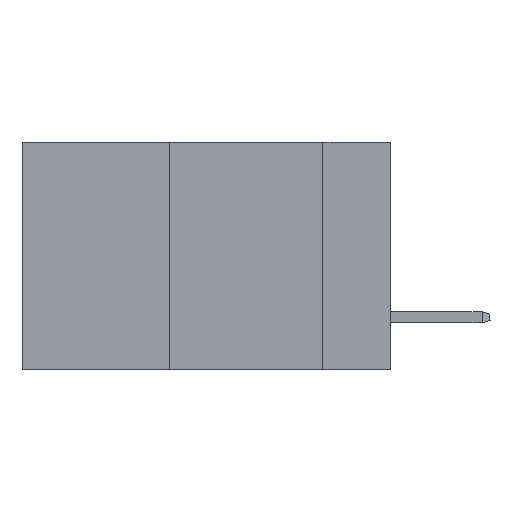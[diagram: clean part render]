
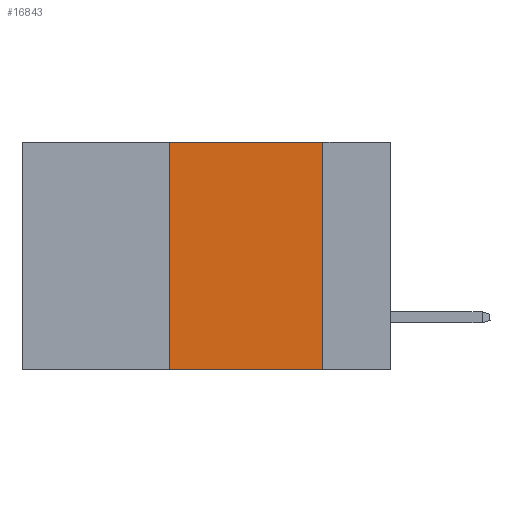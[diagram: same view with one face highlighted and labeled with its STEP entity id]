
A CAD part, left-side view. The second image highlights one B-rep face of the part: STEP entity #16843.
In plain terms, the highlighted planar face has unit normal (-1, 0, 0).
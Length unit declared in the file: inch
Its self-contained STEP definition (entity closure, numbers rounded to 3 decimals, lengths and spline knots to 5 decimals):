
#369 = EDGE_CURVE ( 'NONE', #24583, #14350, #24584, .T. ) ;
#1089 = VERTEX_POINT ( 'NONE', #12770 ) ;
#2658 = DIRECTION ( 'NONE',  ( 1., 0., 0. ) ) ;
#2930 = DIRECTION ( 'NONE',  ( 0., 0., -1. ) ) ;
#3265 = DIRECTION ( 'NONE',  ( 0., 0., 1. ) ) ;
#3415 = EDGE_LOOP ( 'NONE', ( #5046, #25634, #13580, #16845 ) ) ;
#3771 = CARTESIAN_POINT ( 'NONE',  ( 0., 0.6, -0.37 ) ) ;
#5046 = ORIENTED_EDGE ( 'NONE', *, *, #12262, .F. ) ;
#5700 = VECTOR ( 'NONE', #8270, 39.37008 ) ;
#7971 = LINE ( 'NONE', #13589, #9642 ) ;
#8270 = DIRECTION ( 'NONE',  ( 0., -1., 0. ) ) ;
#8736 = FACE_OUTER_BOUND ( 'NONE', #3415, .T. ) ;
#9524 = VERTEX_POINT ( 'NONE', #24870 ) ;
#9642 = VECTOR ( 'NONE', #20105, 39.37008 ) ;
#12262 = EDGE_CURVE ( 'NONE', #14350, #1089, #7971, .T. ) ;
#12770 = CARTESIAN_POINT ( 'NONE',  ( 0., 0.11, -0.37 ) ) ;
#13580 = ORIENTED_EDGE ( 'NONE', *, *, #20589, .F. ) ;
#13589 = CARTESIAN_POINT ( 'NONE',  ( 0., 0.11, 0. ) ) ;
#14350 = VERTEX_POINT ( 'NONE', #20264 ) ;
#15600 = CARTESIAN_POINT ( 'NONE',  ( 0., 0.6, 0. ) ) ;
#15626 = LINE ( 'NONE', #24639, #22579 ) ;
#16843 = ADVANCED_FACE ( 'NONE', ( #8736 ), #25877, .F. ) ;
#16845 = ORIENTED_EDGE ( 'NONE', *, *, #19358, .T. ) ;
#18557 = DIRECTION ( 'NONE',  ( 0., -1., 0. ) ) ;
#18572 = AXIS2_PLACEMENT_3D ( 'NONE', #15600, #2658, #2930 ) ;
#19358 = EDGE_CURVE ( 'NONE', #9524, #1089, #22210, .T. ) ;
#20105 = DIRECTION ( 'NONE',  ( 0., 0., -1. ) ) ;
#20264 = CARTESIAN_POINT ( 'NONE',  ( 0., 0.11, 0. ) ) ;
#20589 = EDGE_CURVE ( 'NONE', #9524, #24583, #15626, .T. ) ;
#20594 = CARTESIAN_POINT ( 'NONE',  ( 0., 0.36, 0. ) ) ;
#22210 = LINE ( 'NONE', #3771, #24174 ) ;
#22579 = VECTOR ( 'NONE', #3265, 39.37008 ) ;
#24174 = VECTOR ( 'NONE', #18557, 39.37008 ) ;
#24583 = VERTEX_POINT ( 'NONE', #20594 ) ;
#24584 = LINE ( 'NONE', #25414, #5700 ) ;
#24639 = CARTESIAN_POINT ( 'NONE',  ( 0., 0.36, 0. ) ) ;
#24870 = CARTESIAN_POINT ( 'NONE',  ( 0., 0.36, -0.37 ) ) ;
#25414 = CARTESIAN_POINT ( 'NONE',  ( 0., 0.6, 0. ) ) ;
#25634 = ORIENTED_EDGE ( 'NONE', *, *, #369, .F. ) ;
#25877 = PLANE ( 'NONE',  #18572 ) ;
